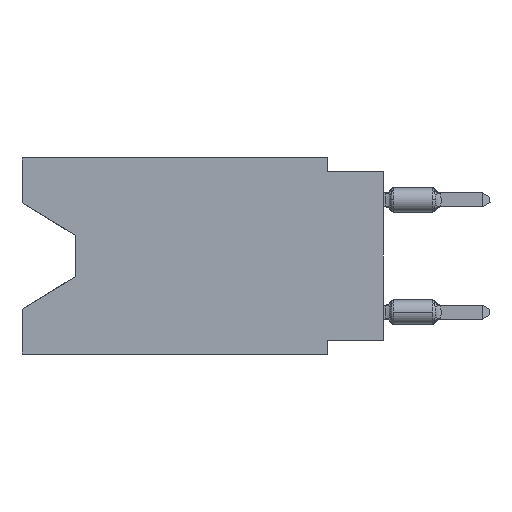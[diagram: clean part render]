
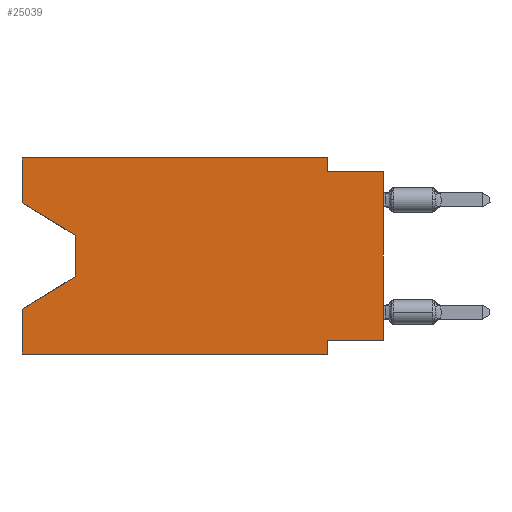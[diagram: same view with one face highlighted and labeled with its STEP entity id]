
A CAD part, left-side view. The second image highlights one B-rep face of the part: STEP entity #25039.
In plain terms, the highlighted planar face has unit normal (-1, 0, 0).
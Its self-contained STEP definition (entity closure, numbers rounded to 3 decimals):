
#99 = DIRECTION ( 'NONE',  ( 0., 0., -1. ) ) ;
#384 = VECTOR ( 'NONE', #1139, 1000. ) ;
#854 = LINE ( 'NONE', #13692, #13166 ) ;
#992 = DIRECTION ( 'NONE',  ( 0., -0.855, -0.519 ) ) ;
#1085 = CARTESIAN_POINT ( 'NONE',  ( 0., 13.97, -5.385 ) ) ;
#1139 = DIRECTION ( 'NONE',  ( 0., 0., 1. ) ) ;
#1164 = VECTOR ( 'NONE', #992, 1000. ) ;
#1743 = CARTESIAN_POINT ( 'NONE',  ( 0., 16.383, -8.89 ) ) ;
#1785 = VERTEX_POINT ( 'NONE', #23734 ) ;
#2057 = EDGE_CURVE ( 'NONE', #4169, #7057, #11947, .T. ) ;
#2104 = EDGE_CURVE ( 'NONE', #26333, #16063, #25288, .T. ) ;
#2109 = ORIENTED_EDGE ( 'NONE', *, *, #10287, .F. ) ;
#3033 = AXIS2_PLACEMENT_3D ( 'NONE', #20334, #20894, #25246 ) ;
#3121 = LINE ( 'NONE', #11862, #384 ) ;
#3492 = ORIENTED_EDGE ( 'NONE', *, *, #5396, .T. ) ;
#3600 = ORIENTED_EDGE ( 'NONE', *, *, #22991, .F. ) ;
#3803 = CARTESIAN_POINT ( 'NONE',  ( 0., 0., -0.635 ) ) ;
#3816 = VECTOR ( 'NONE', #11795, 1000. ) ;
#4169 = VERTEX_POINT ( 'NONE', #6815 ) ;
#4758 = EDGE_CURVE ( 'NONE', #21614, #7057, #854, .T. ) ;
#4814 = LINE ( 'NONE', #21852, #6992 ) ;
#5308 = LINE ( 'NONE', #24453, #8296 ) ;
#5396 = EDGE_CURVE ( 'NONE', #18110, #15181, #18854, .T. ) ;
#5868 = CARTESIAN_POINT ( 'NONE',  ( 0., 16.383, -8.89 ) ) ;
#5871 = CARTESIAN_POINT ( 'NONE',  ( 0., 16.383, -6.852 ) ) ;
#5950 = VERTEX_POINT ( 'NONE', #22378 ) ;
#6815 = CARTESIAN_POINT ( 'NONE',  ( 0., 0., -8.255 ) ) ;
#6987 = EDGE_CURVE ( 'NONE', #1785, #21614, #10302, .T. ) ;
#6990 = DIRECTION ( 'NONE',  ( 0., -1., 0. ) ) ;
#6992 = VECTOR ( 'NONE', #11304, 1000. ) ;
#7057 = VERTEX_POINT ( 'NONE', #3803 ) ;
#7093 = CARTESIAN_POINT ( 'NONE',  ( 0., 16.383, -2.038 ) ) ;
#7580 = DIRECTION ( 'NONE',  ( 0., 0., 1. ) ) ;
#7899 = CARTESIAN_POINT ( 'NONE',  ( 0., 2.54, 0. ) ) ;
#8086 = PLANE ( 'NONE',  #3033 ) ;
#8243 = VECTOR ( 'NONE', #24761, 1000. ) ;
#8296 = VECTOR ( 'NONE', #11934, 1000. ) ;
#9295 = EDGE_CURVE ( 'NONE', #26574, #12791, #4814, .T. ) ;
#10156 = ORIENTED_EDGE ( 'NONE', *, *, #4758, .F. ) ;
#10287 = EDGE_CURVE ( 'NONE', #4169, #5950, #5308, .T. ) ;
#10302 = LINE ( 'NONE', #7899, #23265 ) ;
#10383 = ORIENTED_EDGE ( 'NONE', *, *, #13677, .T. ) ;
#10745 = CARTESIAN_POINT ( 'NONE',  ( 0., 13.97, -3.505 ) ) ;
#11274 = VECTOR ( 'NONE', #25938, 1000. ) ;
#11304 = DIRECTION ( 'NONE',  ( 0., 0., 1. ) ) ;
#11795 = DIRECTION ( 'NONE',  ( 0., -1., 0. ) ) ;
#11862 = CARTESIAN_POINT ( 'NONE',  ( 0., 16.383, 0. ) ) ;
#11931 = VECTOR ( 'NONE', #7580, 1000. ) ;
#11934 = DIRECTION ( 'NONE',  ( 0., 1., 0. ) ) ;
#11947 = LINE ( 'NONE', #16714, #11931 ) ;
#12013 = VECTOR ( 'NONE', #6990, 1000. ) ;
#12791 = VERTEX_POINT ( 'NONE', #20420 ) ;
#12931 = EDGE_CURVE ( 'NONE', #12791, #1785, #13749, .T. ) ;
#13166 = VECTOR ( 'NONE', #21998, 1000. ) ;
#13172 = ORIENTED_EDGE ( 'NONE', *, *, #2057, .T. ) ;
#13298 = CARTESIAN_POINT ( 'NONE',  ( 0., 16.383, -2.038 ) ) ;
#13334 = ORIENTED_EDGE ( 'NONE', *, *, #2104, .T. ) ;
#13677 = EDGE_CURVE ( 'NONE', #20689, #18110, #15063, .T. ) ;
#13692 = CARTESIAN_POINT ( 'NONE',  ( 0., 0., -0.635 ) ) ;
#13749 = LINE ( 'NONE', #17545, #12013 ) ;
#14259 = CARTESIAN_POINT ( 'NONE',  ( 0., 2.54, -0.635 ) ) ;
#14501 = ORIENTED_EDGE ( 'NONE', *, *, #21642, .F. ) ;
#14957 = LINE ( 'NONE', #25785, #11274 ) ;
#15063 = LINE ( 'NONE', #25752, #17406 ) ;
#15181 = VERTEX_POINT ( 'NONE', #5871 ) ;
#15842 = ORIENTED_EDGE ( 'NONE', *, *, #9295, .F. ) ;
#15963 = LINE ( 'NONE', #7093, #1164 ) ;
#16063 = VERTEX_POINT ( 'NONE', #16351 ) ;
#16150 = ORIENTED_EDGE ( 'NONE', *, *, #19313, .T. ) ;
#16351 = CARTESIAN_POINT ( 'NONE',  ( 0., 2.54, -8.89 ) ) ;
#16714 = CARTESIAN_POINT ( 'NONE',  ( 0., 0., 0. ) ) ;
#17256 = ORIENTED_EDGE ( 'NONE', *, *, #12931, .F. ) ;
#17406 = VECTOR ( 'NONE', #99, 1000. ) ;
#17451 = ORIENTED_EDGE ( 'NONE', *, *, #6987, .F. ) ;
#17545 = CARTESIAN_POINT ( 'NONE',  ( 0., 16.383, 0. ) ) ;
#18110 = VERTEX_POINT ( 'NONE', #21390 ) ;
#18641 = FACE_OUTER_BOUND ( 'NONE', #27315, .T. ) ;
#18854 = LINE ( 'NONE', #1085, #8243 ) ;
#19313 = EDGE_CURVE ( 'NONE', #26574, #20689, #15963, .T. ) ;
#20334 = CARTESIAN_POINT ( 'NONE',  ( 0., 16.383, 0. ) ) ;
#20420 = CARTESIAN_POINT ( 'NONE',  ( 0., 16.383, 0. ) ) ;
#20689 = VERTEX_POINT ( 'NONE', #10745 ) ;
#20894 = DIRECTION ( 'NONE',  ( 1., 0., 0. ) ) ;
#21390 = CARTESIAN_POINT ( 'NONE',  ( 0., 13.97, -5.385 ) ) ;
#21614 = VERTEX_POINT ( 'NONE', #14259 ) ;
#21642 = EDGE_CURVE ( 'NONE', #26333, #15181, #3121, .T. ) ;
#21852 = CARTESIAN_POINT ( 'NONE',  ( 0., 16.383, 0. ) ) ;
#21998 = DIRECTION ( 'NONE',  ( 0., -1., 0. ) ) ;
#22378 = CARTESIAN_POINT ( 'NONE',  ( 0., 2.54, -8.255 ) ) ;
#22991 = EDGE_CURVE ( 'NONE', #5950, #16063, #14957, .T. ) ;
#23265 = VECTOR ( 'NONE', #25496, 1000. ) ;
#23734 = CARTESIAN_POINT ( 'NONE',  ( 0., 2.54, 0. ) ) ;
#24453 = CARTESIAN_POINT ( 'NONE',  ( 0., 0., -8.255 ) ) ;
#24761 = DIRECTION ( 'NONE',  ( 0., 0.855, -0.519 ) ) ;
#25039 = ADVANCED_FACE ( 'NONE', ( #18641 ), #8086, .F. ) ;
#25246 = DIRECTION ( 'NONE',  ( 0., 0., -1. ) ) ;
#25288 = LINE ( 'NONE', #5868, #3816 ) ;
#25496 = DIRECTION ( 'NONE',  ( 0., 0., -1. ) ) ;
#25752 = CARTESIAN_POINT ( 'NONE',  ( 0., 13.97, -3.505 ) ) ;
#25785 = CARTESIAN_POINT ( 'NONE',  ( 0., 2.54, -8.89 ) ) ;
#25938 = DIRECTION ( 'NONE',  ( 0., 0., -1. ) ) ;
#26333 = VERTEX_POINT ( 'NONE', #1743 ) ;
#26574 = VERTEX_POINT ( 'NONE', #13298 ) ;
#27315 = EDGE_LOOP ( 'NONE', ( #16150, #10383, #3492, #14501, #13334, #3600, #2109, #13172, #10156, #17451, #17256, #15842 ) ) ;
